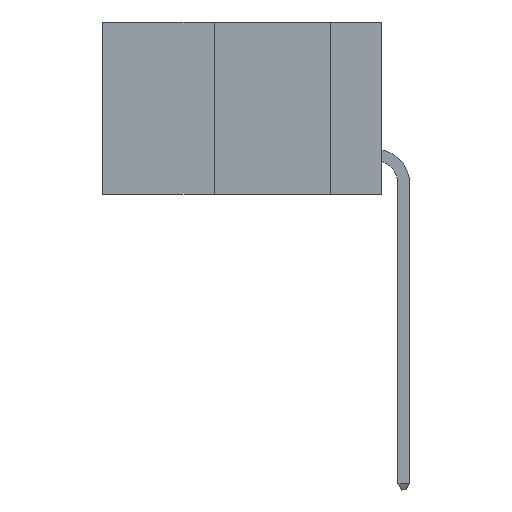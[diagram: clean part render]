
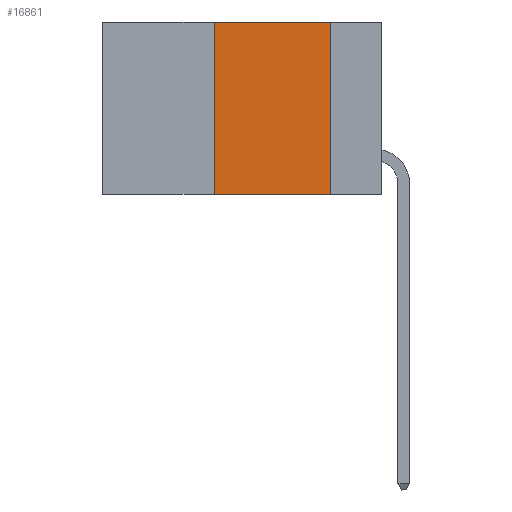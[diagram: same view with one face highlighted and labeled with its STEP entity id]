
A CAD part, left-side view. The second image highlights one B-rep face of the part: STEP entity #16861.
In plain terms, the highlighted planar face has unit normal (-1, 0, 0).
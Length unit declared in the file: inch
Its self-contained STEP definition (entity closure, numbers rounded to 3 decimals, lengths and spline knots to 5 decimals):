
#145 = LINE ( 'NONE', #2420, #18158 ) ;
#566 = CARTESIAN_POINT ( 'NONE',  ( 0., 0.36, 0. ) ) ;
#583 = EDGE_CURVE ( 'NONE', #9478, #15075, #11955, .T. ) ;
#1346 = VECTOR ( 'NONE', #14092, 39.37008 ) ;
#1632 = VERTEX_POINT ( 'NONE', #17697 ) ;
#2420 = CARTESIAN_POINT ( 'NONE',  ( 0., 0.11, 0. ) ) ;
#2484 = EDGE_CURVE ( 'NONE', #7055, #9478, #5394, .T. ) ;
#2788 = CARTESIAN_POINT ( 'NONE',  ( 0., 0.36, 0. ) ) ;
#4251 = ORIENTED_EDGE ( 'NONE', *, *, #16912, .F. ) ;
#4462 = DIRECTION ( 'NONE',  ( 0., -1., 0. ) ) ;
#5380 = DIRECTION ( 'NONE',  ( 1., 0., 0. ) ) ;
#5394 = LINE ( 'NONE', #566, #1346 ) ;
#5726 = CARTESIAN_POINT ( 'NONE',  ( 0., 0.36, -0.37 ) ) ;
#6251 = VECTOR ( 'NONE', #19098, 39.37008 ) ;
#6513 = ORIENTED_EDGE ( 'NONE', *, *, #583, .F. ) ;
#7055 = VERTEX_POINT ( 'NONE', #5726 ) ;
#7212 = DIRECTION ( 'NONE',  ( 0., 0., -1. ) ) ;
#8011 = LINE ( 'NONE', #11276, #6251 ) ;
#8666 = CARTESIAN_POINT ( 'NONE',  ( 0., 0.6, 0. ) ) ;
#9478 = VERTEX_POINT ( 'NONE', #2788 ) ;
#11276 = CARTESIAN_POINT ( 'NONE',  ( 0., 0.6, -0.37 ) ) ;
#11812 = PLANE ( 'NONE',  #17233 ) ;
#11955 = LINE ( 'NONE', #20380, #17190 ) ;
#11956 = DIRECTION ( 'NONE',  ( 0., 0., -1. ) ) ;
#14092 = DIRECTION ( 'NONE',  ( 0., 0., 1. ) ) ;
#14935 = FACE_OUTER_BOUND ( 'NONE', #18742, .T. ) ;
#15075 = VERTEX_POINT ( 'NONE', #19559 ) ;
#15322 = ORIENTED_EDGE ( 'NONE', *, *, #2484, .F. ) ;
#16333 = ORIENTED_EDGE ( 'NONE', *, *, #18043, .T. ) ;
#16861 = ADVANCED_FACE ( 'NONE', ( #14935 ), #11812, .F. ) ;
#16912 = EDGE_CURVE ( 'NONE', #15075, #1632, #145, .T. ) ;
#17190 = VECTOR ( 'NONE', #4462, 39.37008 ) ;
#17233 = AXIS2_PLACEMENT_3D ( 'NONE', #8666, #5380, #7212 ) ;
#17697 = CARTESIAN_POINT ( 'NONE',  ( 0., 0.11, -0.37 ) ) ;
#18043 = EDGE_CURVE ( 'NONE', #7055, #1632, #8011, .T. ) ;
#18158 = VECTOR ( 'NONE', #11956, 39.37008 ) ;
#18742 = EDGE_LOOP ( 'NONE', ( #4251, #6513, #15322, #16333 ) ) ;
#19098 = DIRECTION ( 'NONE',  ( 0., -1., 0. ) ) ;
#19559 = CARTESIAN_POINT ( 'NONE',  ( 0., 0.11, 0. ) ) ;
#20380 = CARTESIAN_POINT ( 'NONE',  ( 0., 0.6, 0. ) ) ;
